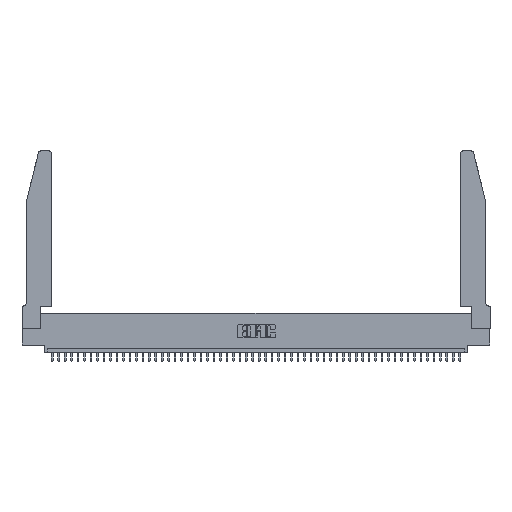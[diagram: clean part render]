
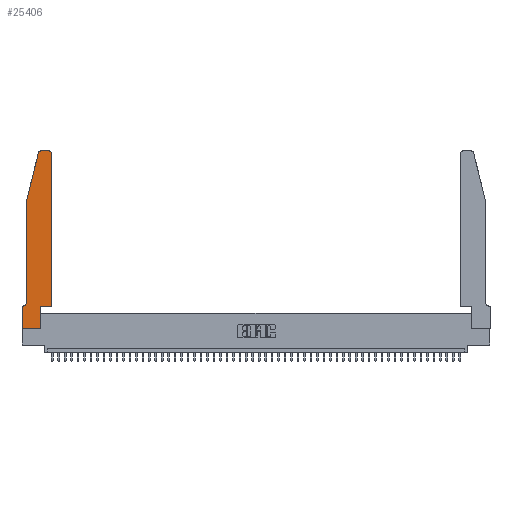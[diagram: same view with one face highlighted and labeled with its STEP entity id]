
A CAD part, top view. The second image highlights one B-rep face of the part: STEP entity #25406.
In plain terms, the highlighted planar face has unit normal (0, 0, 1).
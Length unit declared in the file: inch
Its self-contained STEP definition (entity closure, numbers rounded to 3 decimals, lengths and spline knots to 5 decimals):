
#1396 = DIRECTION ( 'NONE',  ( 0., 0., 1. ) ) ;
#1861 = ORIENTED_EDGE ( 'NONE', *, *, #21106, .T. ) ;
#4105 = VERTEX_POINT ( 'NONE', #47790 ) ;
#4322 = LINE ( 'NONE', #35592, #41824 ) ;
#4399 = CIRCLE ( 'NONE', #14152, 0.07 ) ;
#5333 = DIRECTION ( 'NONE',  ( 0., -1., 0. ) ) ;
#6005 = CARTESIAN_POINT ( 'NONE',  ( 0.0755, 2., 0.37 ) ) ;
#6076 = VERTEX_POINT ( 'NONE', #6005 ) ;
#6751 = DIRECTION ( 'NONE',  ( -0.239, -0.971, 0. ) ) ;
#6763 = VERTEX_POINT ( 'NONE', #40303 ) ;
#7467 = DIRECTION ( 'NONE',  ( 0., 0., -1. ) ) ;
#8149 = CARTESIAN_POINT ( 'NONE',  ( 0.284, 2.72, 0.37 ) ) ;
#8485 = ORIENTED_EDGE ( 'NONE', *, *, #33386, .T. ) ;
#8496 = EDGE_CURVE ( 'NONE', #42637, #47489, #4322, .T. ) ;
#10202 = ORIENTED_EDGE ( 'NONE', *, *, #23973, .T. ) ;
#10423 = EDGE_CURVE ( 'NONE', #47489, #6763, #31980, .T. ) ;
#10447 = VECTOR ( 'NONE', #6751, 39.37008 ) ;
#11542 = CARTESIAN_POINT ( 'NONE',  ( 0.0055, 0.42, 0.37 ) ) ;
#11594 = CARTESIAN_POINT ( 'NONE',  ( 0.2865, 0.35, 0.37 ) ) ;
#11946 = CARTESIAN_POINT ( 'NONE',  ( 0., 0.35, 0.37 ) ) ;
#13255 = VECTOR ( 'NONE', #13499, 39.37008 ) ;
#13499 = DIRECTION ( 'NONE',  ( -1., 0., 0. ) ) ;
#13929 = AXIS2_PLACEMENT_3D ( 'NONE', #8149, #46992, #23570 ) ;
#14152 = AXIS2_PLACEMENT_3D ( 'NONE', #11542, #7467, #46328 ) ;
#14349 = ORIENTED_EDGE ( 'NONE', *, *, #14468, .T. ) ;
#14468 = EDGE_CURVE ( 'NONE', #39165, #6076, #47924, .T. ) ;
#14858 = AXIS2_PLACEMENT_3D ( 'NONE', #44013, #1396, #24271 ) ;
#15215 = DIRECTION ( 'NONE',  ( 0., -1., 0. ) ) ;
#15674 = VERTEX_POINT ( 'NONE', #11594 ) ;
#15683 = VERTEX_POINT ( 'NONE', #15810 ) ;
#15810 = CARTESIAN_POINT ( 'NONE',  ( 0.284, 2.75, 0.37 ) ) ;
#16178 = LINE ( 'NONE', #19199, #17413 ) ;
#16348 = ORIENTED_EDGE ( 'NONE', *, *, #34345, .T. ) ;
#16875 = VERTEX_POINT ( 'NONE', #31762 ) ;
#17140 = AXIS2_PLACEMENT_3D ( 'NONE', #11946, #34467, #46563 ) ;
#17261 = CARTESIAN_POINT ( 'NONE',  ( 0.0755, 0.35, 0.37 ) ) ;
#17413 = VECTOR ( 'NONE', #34423, 39.37008 ) ;
#17681 = CARTESIAN_POINT ( 'NONE',  ( 0.0755, 2., 0.37 ) ) ;
#18604 = ORIENTED_EDGE ( 'NONE', *, *, #29182, .T. ) ;
#19019 = LINE ( 'NONE', #35996, #26852 ) ;
#19199 = CARTESIAN_POINT ( 'NONE',  ( 0.2865, 0.35, 0.37 ) ) ;
#20010 = LINE ( 'NONE', #23182, #38721 ) ;
#20459 = DIRECTION ( 'NONE',  ( -1., 0., 0. ) ) ;
#21106 = EDGE_CURVE ( 'NONE', #15674, #42637, #33255, .T. ) ;
#21241 = CARTESIAN_POINT ( 'NONE',  ( 0.2865, 0., 0.37 ) ) ;
#23182 = CARTESIAN_POINT ( 'NONE',  ( 0., 0., 0.37 ) ) ;
#23570 = DIRECTION ( 'NONE',  ( 1., 0., 0. ) ) ;
#23859 = VECTOR ( 'NONE', #32836, 39.37008 ) ;
#23973 = EDGE_CURVE ( 'NONE', #6076, #37992, #26245, .T. ) ;
#24271 = DIRECTION ( 'NONE',  ( 1., 0., 0. ) ) ;
#25406 = ADVANCED_FACE ( 'NONE', ( #45415 ), #31051, .T. ) ;
#25719 = ORIENTED_EDGE ( 'NONE', *, *, #8496, .T. ) ;
#26245 = LINE ( 'NONE', #17681, #41978 ) ;
#26852 = VECTOR ( 'NONE', #20459, 39.37008 ) ;
#27966 = EDGE_LOOP ( 'NONE', ( #8485, #40252, #14349, #10202, #16348, #36736, #40313, #38355, #18604, #1861, #25719, #28449 ) ) ;
#28200 = CARTESIAN_POINT ( 'NONE',  ( 0.0755, 0.42, 0.37 ) ) ;
#28217 = EDGE_CURVE ( 'NONE', #4105, #30026, #42886, .T. ) ;
#28323 = CARTESIAN_POINT ( 'NONE',  ( 0., 0.35, 0.37 ) ) ;
#28449 = ORIENTED_EDGE ( 'NONE', *, *, #10423, .T. ) ;
#29182 = EDGE_CURVE ( 'NONE', #34011, #15674, #16178, .T. ) ;
#29936 = CARTESIAN_POINT ( 'NONE',  ( 0.0755, 2., 0.37 ) ) ;
#30026 = VERTEX_POINT ( 'NONE', #28323 ) ;
#30697 = EDGE_CURVE ( 'NONE', #16875, #34011, #49238, .T. ) ;
#31051 = PLANE ( 'NONE',  #17140 ) ;
#31762 = CARTESIAN_POINT ( 'NONE',  ( 0., 0., 0.37 ) ) ;
#31980 = CIRCLE ( 'NONE', #14858, 0.03 ) ;
#32836 = DIRECTION ( 'NONE',  ( 1., 0., 0. ) ) ;
#33255 = LINE ( 'NONE', #34647, #39294 ) ;
#33386 = EDGE_CURVE ( 'NONE', #6763, #15683, #19019, .T. ) ;
#34011 = VERTEX_POINT ( 'NONE', #21241 ) ;
#34345 = EDGE_CURVE ( 'NONE', #37992, #4105, #4399, .T. ) ;
#34423 = DIRECTION ( 'NONE',  ( 0., 1., 0. ) ) ;
#34467 = DIRECTION ( 'NONE',  ( 0., 0., 1. ) ) ;
#34647 = CARTESIAN_POINT ( 'NONE',  ( 0.4505, 0.35, 0.37 ) ) ;
#34694 = CARTESIAN_POINT ( 'NONE',  ( 0.25487, 2.72718, 0.37 ) ) ;
#35592 = CARTESIAN_POINT ( 'NONE',  ( 0.4505, 0.35, 0.37 ) ) ;
#35996 = CARTESIAN_POINT ( 'NONE',  ( 0.2605, 2.75, 0.37 ) ) ;
#36736 = ORIENTED_EDGE ( 'NONE', *, *, #28217, .T. ) ;
#37806 = CARTESIAN_POINT ( 'NONE',  ( 0.4505, 2.72, 0.37 ) ) ;
#37992 = VERTEX_POINT ( 'NONE', #28200 ) ;
#38355 = ORIENTED_EDGE ( 'NONE', *, *, #30697, .T. ) ;
#38721 = VECTOR ( 'NONE', #15215, 39.37008 ) ;
#38802 = EDGE_CURVE ( 'NONE', #15683, #39165, #49672, .T. ) ;
#39165 = VERTEX_POINT ( 'NONE', #34694 ) ;
#39294 = VECTOR ( 'NONE', #49483, 39.37008 ) ;
#39814 = DIRECTION ( 'NONE',  ( 0., 1., 0. ) ) ;
#40157 = CARTESIAN_POINT ( 'NONE',  ( 0.4505, 0.35, 0.37 ) ) ;
#40252 = ORIENTED_EDGE ( 'NONE', *, *, #38802, .T. ) ;
#40303 = CARTESIAN_POINT ( 'NONE',  ( 0.4205, 2.75, 0.37 ) ) ;
#40313 = ORIENTED_EDGE ( 'NONE', *, *, #45489, .T. ) ;
#40767 = CARTESIAN_POINT ( 'NONE',  ( 0., 0., 0.37 ) ) ;
#41824 = VECTOR ( 'NONE', #39814, 39.37008 ) ;
#41978 = VECTOR ( 'NONE', #5333, 39.37008 ) ;
#42637 = VERTEX_POINT ( 'NONE', #40157 ) ;
#42886 = LINE ( 'NONE', #17261, #13255 ) ;
#44013 = CARTESIAN_POINT ( 'NONE',  ( 0.4205, 2.72, 0.37 ) ) ;
#45415 = FACE_OUTER_BOUND ( 'NONE', #27966, .T. ) ;
#45489 = EDGE_CURVE ( 'NONE', #30026, #16875, #20010, .T. ) ;
#46328 = DIRECTION ( 'NONE',  ( -1., 0., 0. ) ) ;
#46563 = DIRECTION ( 'NONE',  ( 1., 0., 0. ) ) ;
#46992 = DIRECTION ( 'NONE',  ( 0., 0., 1. ) ) ;
#47489 = VERTEX_POINT ( 'NONE', #37806 ) ;
#47790 = CARTESIAN_POINT ( 'NONE',  ( 0.0055, 0.35, 0.37 ) ) ;
#47924 = LINE ( 'NONE', #29936, #10447 ) ;
#49238 = LINE ( 'NONE', #40767, #23859 ) ;
#49483 = DIRECTION ( 'NONE',  ( 1., 0., 0. ) ) ;
#49672 = CIRCLE ( 'NONE', #13929, 0.03 ) ;
